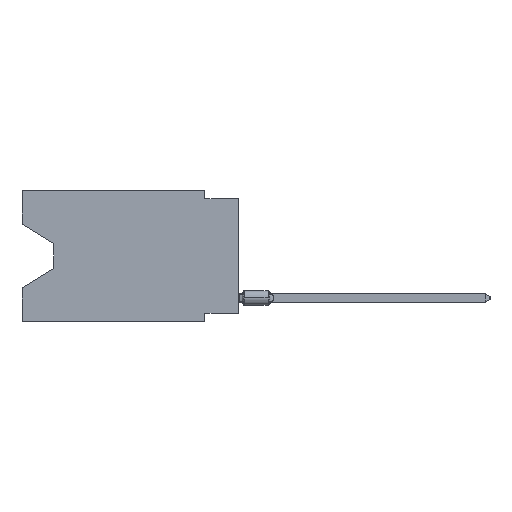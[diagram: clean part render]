
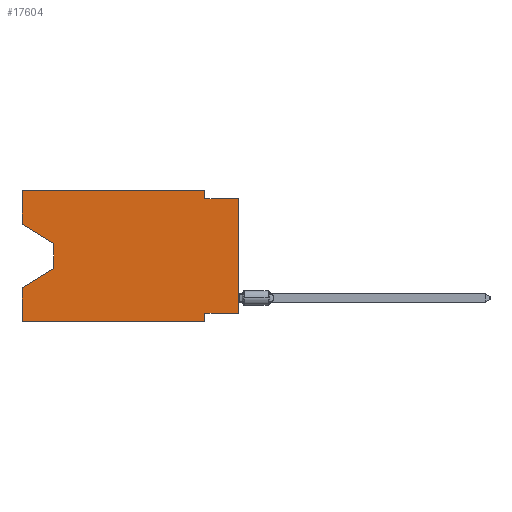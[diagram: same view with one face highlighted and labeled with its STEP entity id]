
A CAD part, left-side view. The second image highlights one B-rep face of the part: STEP entity #17604.
In plain terms, the highlighted planar face has unit normal (-1, 0, 0).
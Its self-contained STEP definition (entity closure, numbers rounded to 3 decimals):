
#2207 = ORIENTED_EDGE ( 'NONE', *, *, #31894, .F. ) ;
#3427 = CARTESIAN_POINT ( 'NONE',  ( 0., 2.54, -9.906 ) ) ;
#4056 = VECTOR ( 'NONE', #13551, 1000. ) ;
#4206 = CARTESIAN_POINT ( 'NONE',  ( 0., 0., 0. ) ) ;
#4983 = EDGE_CURVE ( 'NONE', #31481, #63008, #19425, .T. ) ;
#5651 = LINE ( 'NONE', #18935, #29705 ) ;
#5685 = CARTESIAN_POINT ( 'NONE',  ( 0., 2.54, -9.271 ) ) ;
#6858 = DIRECTION ( 'NONE',  ( 0., -1., 0. ) ) ;
#6990 = CARTESIAN_POINT ( 'NONE',  ( 0., 13.97, -5.893 ) ) ;
#7511 = EDGE_LOOP ( 'NONE', ( #65089, #21169, #55228, #21005, #33956, #74670, #2207, #70398, #60608, #67464, #70213, #50848 ) ) ;
#7760 = VERTEX_POINT ( 'NONE', #51764 ) ;
#7796 = DIRECTION ( 'NONE',  ( 0., 0., -1. ) ) ;
#9413 = VERTEX_POINT ( 'NONE', #40724 ) ;
#10088 = CARTESIAN_POINT ( 'NONE',  ( 0., 13.97, -4.013 ) ) ;
#11655 = CARTESIAN_POINT ( 'NONE',  ( 0., 16.383, -9.906 ) ) ;
#12960 = CARTESIAN_POINT ( 'NONE',  ( 0., 2.54, 0. ) ) ;
#13551 = DIRECTION ( 'NONE',  ( 0., 0., 1. ) ) ;
#14099 = VECTOR ( 'NONE', #74382, 1000. ) ;
#14939 = VERTEX_POINT ( 'NONE', #5685 ) ;
#15068 = EDGE_CURVE ( 'NONE', #48229, #7760, #47086, .T. ) ;
#15946 = DIRECTION ( 'NONE',  ( 0., 0., 1. ) ) ;
#16618 = VECTOR ( 'NONE', #52705, 1000. ) ;
#17293 = CARTESIAN_POINT ( 'NONE',  ( 0., 16.383, -9.906 ) ) ;
#17604 = ADVANCED_FACE ( 'NONE', ( #30808 ), #25720, .F. ) ;
#18935 = CARTESIAN_POINT ( 'NONE',  ( 0., 13.97, -4.013 ) ) ;
#19425 = LINE ( 'NONE', #38934, #4056 ) ;
#20176 = AXIS2_PLACEMENT_3D ( 'NONE', #31577, #60826, #49527 ) ;
#21005 = ORIENTED_EDGE ( 'NONE', *, *, #4983, .F. ) ;
#21026 = LINE ( 'NONE', #4206, #49074 ) ;
#21169 = ORIENTED_EDGE ( 'NONE', *, *, #40807, .T. ) ;
#23814 = VERTEX_POINT ( 'NONE', #30781 ) ;
#23839 = LINE ( 'NONE', #72211, #75338 ) ;
#25088 = VERTEX_POINT ( 'NONE', #3427 ) ;
#25226 = LINE ( 'NONE', #49026, #62763 ) ;
#25720 = PLANE ( 'NONE',  #20176 ) ;
#26768 = DIRECTION ( 'NONE',  ( 0., -1., 0. ) ) ;
#28043 = EDGE_CURVE ( 'NONE', #31481, #25088, #49131, .T. ) ;
#29705 = VECTOR ( 'NONE', #41979, 1000. ) ;
#29773 = EDGE_CURVE ( 'NONE', #9413, #50076, #50606, .T. ) ;
#30781 = CARTESIAN_POINT ( 'NONE',  ( 0., 13.97, -5.893 ) ) ;
#30808 = FACE_OUTER_BOUND ( 'NONE', #7511, .T. ) ;
#31481 = VERTEX_POINT ( 'NONE', #17293 ) ;
#31577 = CARTESIAN_POINT ( 'NONE',  ( 0., 16.383, 0. ) ) ;
#31894 = EDGE_CURVE ( 'NONE', #64535, #14939, #47529, .T. ) ;
#32168 = EDGE_CURVE ( 'NONE', #23814, #63008, #76840, .T. ) ;
#33943 = VECTOR ( 'NONE', #73417, 1000. ) ;
#33956 = ORIENTED_EDGE ( 'NONE', *, *, #28043, .T. ) ;
#35821 = CARTESIAN_POINT ( 'NONE',  ( 0., 0., -9.271 ) ) ;
#38934 = CARTESIAN_POINT ( 'NONE',  ( 0., 16.383, 0. ) ) ;
#40190 = EDGE_CURVE ( 'NONE', #9413, #48229, #44087, .T. ) ;
#40724 = CARTESIAN_POINT ( 'NONE',  ( 0., 16.383, -2.546 ) ) ;
#40807 = EDGE_CURVE ( 'NONE', #50076, #23814, #5651, .T. ) ;
#41979 = DIRECTION ( 'NONE',  ( 0., 0., -1. ) ) ;
#44087 = LINE ( 'NONE', #69029, #67136 ) ;
#47086 = LINE ( 'NONE', #71253, #61046 ) ;
#47529 = LINE ( 'NONE', #35821, #76401 ) ;
#48229 = VERTEX_POINT ( 'NONE', #54714 ) ;
#49026 = CARTESIAN_POINT ( 'NONE',  ( 0., 0., -0.635 ) ) ;
#49074 = VECTOR ( 'NONE', #15946, 1000. ) ;
#49131 = LINE ( 'NONE', #11655, #70045 ) ;
#49527 = DIRECTION ( 'NONE',  ( 0., 0., -1. ) ) ;
#50076 = VERTEX_POINT ( 'NONE', #10088 ) ;
#50606 = LINE ( 'NONE', #67751, #14099 ) ;
#50848 = ORIENTED_EDGE ( 'NONE', *, *, #40190, .F. ) ;
#51764 = CARTESIAN_POINT ( 'NONE',  ( 0., 2.54, 0. ) ) ;
#52705 = DIRECTION ( 'NONE',  ( 0., 0.855, -0.519 ) ) ;
#54158 = DIRECTION ( 'NONE',  ( 0., 1., 0. ) ) ;
#54714 = CARTESIAN_POINT ( 'NONE',  ( 0., 16.383, 0. ) ) ;
#55228 = ORIENTED_EDGE ( 'NONE', *, *, #32168, .T. ) ;
#55865 = LINE ( 'NONE', #12960, #33943 ) ;
#56346 = CARTESIAN_POINT ( 'NONE',  ( 0., 0., -0.635 ) ) ;
#56550 = DIRECTION ( 'NONE',  ( 0., 0., 1. ) ) ;
#57383 = CARTESIAN_POINT ( 'NONE',  ( 0., 2.54, -0.635 ) ) ;
#59048 = VERTEX_POINT ( 'NONE', #56346 ) ;
#60608 = ORIENTED_EDGE ( 'NONE', *, *, #64351, .F. ) ;
#60826 = DIRECTION ( 'NONE',  ( 1., 0., 0. ) ) ;
#61046 = VECTOR ( 'NONE', #6858, 1000. ) ;
#62650 = CARTESIAN_POINT ( 'NONE',  ( 0., 16.383, -7.36 ) ) ;
#62763 = VECTOR ( 'NONE', #26768, 1000. ) ;
#63008 = VERTEX_POINT ( 'NONE', #62650 ) ;
#64351 = EDGE_CURVE ( 'NONE', #75915, #59048, #25226, .T. ) ;
#64535 = VERTEX_POINT ( 'NONE', #70422 ) ;
#65089 = ORIENTED_EDGE ( 'NONE', *, *, #29773, .T. ) ;
#67136 = VECTOR ( 'NONE', #56550, 1000. ) ;
#67371 = EDGE_CURVE ( 'NONE', #14939, #25088, #23839, .T. ) ;
#67464 = ORIENTED_EDGE ( 'NONE', *, *, #72415, .F. ) ;
#67751 = CARTESIAN_POINT ( 'NONE',  ( 0., 16.383, -2.546 ) ) ;
#69029 = CARTESIAN_POINT ( 'NONE',  ( 0., 16.383, 0. ) ) ;
#70045 = VECTOR ( 'NONE', #74463, 1000. ) ;
#70213 = ORIENTED_EDGE ( 'NONE', *, *, #15068, .F. ) ;
#70398 = ORIENTED_EDGE ( 'NONE', *, *, #76341, .T. ) ;
#70422 = CARTESIAN_POINT ( 'NONE',  ( 0., 0., -9.271 ) ) ;
#71253 = CARTESIAN_POINT ( 'NONE',  ( 0., 16.383, 0. ) ) ;
#72211 = CARTESIAN_POINT ( 'NONE',  ( 0., 2.54, -9.906 ) ) ;
#72415 = EDGE_CURVE ( 'NONE', #7760, #75915, #55865, .T. ) ;
#73417 = DIRECTION ( 'NONE',  ( 0., 0., -1. ) ) ;
#74382 = DIRECTION ( 'NONE',  ( 0., -0.855, -0.519 ) ) ;
#74463 = DIRECTION ( 'NONE',  ( 0., -1., 0. ) ) ;
#74670 = ORIENTED_EDGE ( 'NONE', *, *, #67371, .F. ) ;
#75338 = VECTOR ( 'NONE', #7796, 1000. ) ;
#75915 = VERTEX_POINT ( 'NONE', #57383 ) ;
#76341 = EDGE_CURVE ( 'NONE', #64535, #59048, #21026, .T. ) ;
#76401 = VECTOR ( 'NONE', #54158, 1000. ) ;
#76840 = LINE ( 'NONE', #6990, #16618 ) ;
